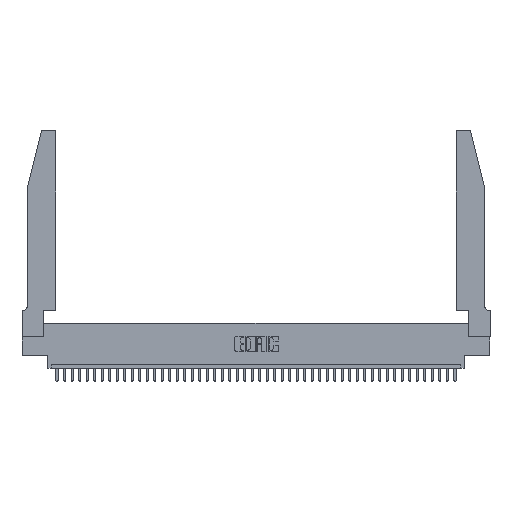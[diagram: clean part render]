
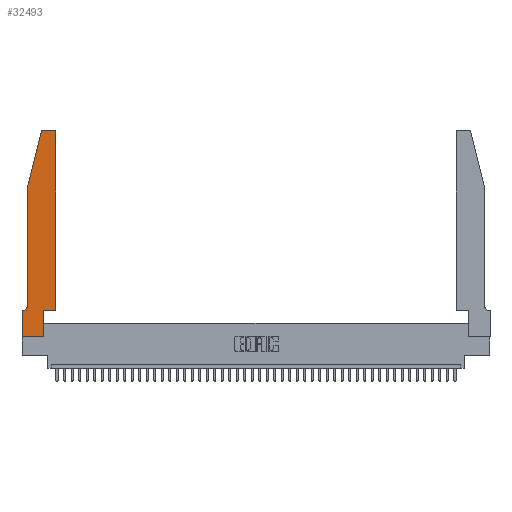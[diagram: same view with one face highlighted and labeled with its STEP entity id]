
A CAD part, top view. The second image highlights one B-rep face of the part: STEP entity #32493.
In plain terms, the highlighted planar face has unit normal (0, 0, 1).
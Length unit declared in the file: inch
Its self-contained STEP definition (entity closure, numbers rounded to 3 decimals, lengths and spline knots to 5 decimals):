
#1047 = CARTESIAN_POINT ( 'NONE',  ( 0.0755, 2., 0.37 ) ) ;
#1099 = VECTOR ( 'NONE', #38962, 39.37008 ) ;
#1119 = FACE_OUTER_BOUND ( 'NONE', #25102, .T. ) ;
#1411 = EDGE_CURVE ( 'NONE', #17696, #33769, #24357, .T. ) ;
#1927 = LINE ( 'NONE', #16082, #43422 ) ;
#2068 = VECTOR ( 'NONE', #18212, 39.37008 ) ;
#2736 = CIRCLE ( 'NONE', #26827, 0.03 ) ;
#2953 = VERTEX_POINT ( 'NONE', #4445 ) ;
#3896 = LINE ( 'NONE', #5352, #18376 ) ;
#4217 = EDGE_CURVE ( 'NONE', #33769, #29964, #24184, .T. ) ;
#4397 = EDGE_CURVE ( 'NONE', #36205, #2953, #17223, .T. ) ;
#4445 = CARTESIAN_POINT ( 'NONE',  ( 0.4205, 2.75, 0.37 ) ) ;
#4448 = DIRECTION ( 'NONE',  ( -1., 0., 0. ) ) ;
#4806 = CARTESIAN_POINT ( 'NONE',  ( 0., 0., 0.37 ) ) ;
#5143 = ORIENTED_EDGE ( 'NONE', *, *, #42124, .T. ) ;
#5352 = CARTESIAN_POINT ( 'NONE',  ( 0.4505, 0.35, 0.37 ) ) ;
#5891 = EDGE_CURVE ( 'NONE', #28611, #9246, #10174, .T. ) ;
#6174 = DIRECTION ( 'NONE',  ( 0., 1., 0. ) ) ;
#7845 = CARTESIAN_POINT ( 'NONE',  ( 0.4205, 2.72, 0.37 ) ) ;
#9045 = DIRECTION ( 'NONE',  ( 0., 0., 1. ) ) ;
#9246 = VERTEX_POINT ( 'NONE', #1047 ) ;
#9810 = AXIS2_PLACEMENT_3D ( 'NONE', #7845, #14760, #38531 ) ;
#10054 = ORIENTED_EDGE ( 'NONE', *, *, #1411, .T. ) ;
#10174 = LINE ( 'NONE', #28680, #30915 ) ;
#11114 = LINE ( 'NONE', #15453, #2068 ) ;
#11143 = CARTESIAN_POINT ( 'NONE',  ( 0., 0., 0.37 ) ) ;
#11722 = VECTOR ( 'NONE', #35917, 39.37008 ) ;
#14369 = DIRECTION ( 'NONE',  ( 1., 0., 0. ) ) ;
#14527 = AXIS2_PLACEMENT_3D ( 'NONE', #43108, #9045, #33290 ) ;
#14609 = ORIENTED_EDGE ( 'NONE', *, *, #4397, .T. ) ;
#14760 = DIRECTION ( 'NONE',  ( 0., 0., 1. ) ) ;
#15453 = CARTESIAN_POINT ( 'NONE',  ( 0., 0., 0.37 ) ) ;
#16082 = CARTESIAN_POINT ( 'NONE',  ( 0.2865, 0.35, 0.37 ) ) ;
#16674 = CARTESIAN_POINT ( 'NONE',  ( 0.0055, 0.35, 0.37 ) ) ;
#17223 = CIRCLE ( 'NONE', #9810, 0.03 ) ;
#17302 = EDGE_CURVE ( 'NONE', #2953, #28979, #42153, .T. ) ;
#17434 = ORIENTED_EDGE ( 'NONE', *, *, #34418, .T. ) ;
#17696 = VERTEX_POINT ( 'NONE', #31100 ) ;
#18212 = DIRECTION ( 'NONE',  ( 1., 0., 0. ) ) ;
#18376 = VECTOR ( 'NONE', #19092, 39.37008 ) ;
#19009 = DIRECTION ( 'NONE',  ( -1., 0., 0. ) ) ;
#19092 = DIRECTION ( 'NONE',  ( 0., 1., 0. ) ) ;
#19240 = EDGE_CURVE ( 'NONE', #21000, #33388, #11114, .T. ) ;
#19269 = VERTEX_POINT ( 'NONE', #37782 ) ;
#19767 = PLANE ( 'NONE',  #14527 ) ;
#20095 = CARTESIAN_POINT ( 'NONE',  ( 0.2865, 0.35, 0.37 ) ) ;
#20472 = DIRECTION ( 'NONE',  ( 1., 0., 0. ) ) ;
#20912 = CARTESIAN_POINT ( 'NONE',  ( 0.4505, 0.35, 0.37 ) ) ;
#21000 = VERTEX_POINT ( 'NONE', #4806 ) ;
#21328 = CARTESIAN_POINT ( 'NONE',  ( 0., 0.35, 0.37 ) ) ;
#22362 = CARTESIAN_POINT ( 'NONE',  ( 0.2605, 2.75, 0.37 ) ) ;
#22455 = CARTESIAN_POINT ( 'NONE',  ( 0.0755, 0.35, 0.37 ) ) ;
#23113 = ORIENTED_EDGE ( 'NONE', *, *, #42888, .T. ) ;
#23360 = VECTOR ( 'NONE', #14369, 39.37008 ) ;
#23473 = LINE ( 'NONE', #32483, #11722 ) ;
#23914 = CARTESIAN_POINT ( 'NONE',  ( 0.4505, 2.72, 0.37 ) ) ;
#24184 = LINE ( 'NONE', #22455, #42802 ) ;
#24357 = CIRCLE ( 'NONE', #38618, 0.07 ) ;
#24699 = CARTESIAN_POINT ( 'NONE',  ( 0.2865, 0., 0.37 ) ) ;
#24901 = CARTESIAN_POINT ( 'NONE',  ( 0.0055, 0.42, 0.37 ) ) ;
#25102 = EDGE_LOOP ( 'NONE', ( #42852, #31682, #36354, #23113, #10054, #36362, #5143, #40101, #42483, #17434, #35818, #14609 ) ) ;
#25788 = DIRECTION ( 'NONE',  ( -1., 0., 0. ) ) ;
#26827 = AXIS2_PLACEMENT_3D ( 'NONE', #43818, #40810, #20472 ) ;
#27795 = VECTOR ( 'NONE', #25788, 39.37008 ) ;
#28123 = CARTESIAN_POINT ( 'NONE',  ( 0.284, 2.75, 0.37 ) ) ;
#28611 = VERTEX_POINT ( 'NONE', #36499 ) ;
#28680 = CARTESIAN_POINT ( 'NONE',  ( 0.0755, 2., 0.37 ) ) ;
#28979 = VERTEX_POINT ( 'NONE', #28123 ) ;
#29964 = VERTEX_POINT ( 'NONE', #21328 ) ;
#30721 = LINE ( 'NONE', #20912, #23360 ) ;
#30915 = VECTOR ( 'NONE', #42482, 39.37008 ) ;
#31100 = CARTESIAN_POINT ( 'NONE',  ( 0.0755, 0.42, 0.37 ) ) ;
#31682 = ORIENTED_EDGE ( 'NONE', *, *, #32652, .T. ) ;
#32483 = CARTESIAN_POINT ( 'NONE',  ( 0.0755, 2., 0.37 ) ) ;
#32493 = ADVANCED_FACE ( 'NONE', ( #1119 ), #19767, .T. ) ;
#32652 = EDGE_CURVE ( 'NONE', #28979, #28611, #2736, .T. ) ;
#33290 = DIRECTION ( 'NONE',  ( 1., 0., 0. ) ) ;
#33388 = VERTEX_POINT ( 'NONE', #24699 ) ;
#33769 = VERTEX_POINT ( 'NONE', #16674 ) ;
#34124 = LINE ( 'NONE', #11143, #1099 ) ;
#34418 = EDGE_CURVE ( 'NONE', #42627, #19269, #30721, .T. ) ;
#35818 = ORIENTED_EDGE ( 'NONE', *, *, #36910, .T. ) ;
#35917 = DIRECTION ( 'NONE',  ( 0., -1., 0. ) ) ;
#36205 = VERTEX_POINT ( 'NONE', #23914 ) ;
#36354 = ORIENTED_EDGE ( 'NONE', *, *, #5891, .T. ) ;
#36362 = ORIENTED_EDGE ( 'NONE', *, *, #4217, .T. ) ;
#36499 = CARTESIAN_POINT ( 'NONE',  ( 0.25487, 2.72718, 0.37 ) ) ;
#36910 = EDGE_CURVE ( 'NONE', #19269, #36205, #3896, .T. ) ;
#37782 = CARTESIAN_POINT ( 'NONE',  ( 0.4505, 0.35, 0.37 ) ) ;
#38531 = DIRECTION ( 'NONE',  ( 1., 0., 0. ) ) ;
#38618 = AXIS2_PLACEMENT_3D ( 'NONE', #24901, #41384, #4448 ) ;
#38850 = EDGE_CURVE ( 'NONE', #33388, #42627, #1927, .T. ) ;
#38962 = DIRECTION ( 'NONE',  ( 0., -1., 0. ) ) ;
#40101 = ORIENTED_EDGE ( 'NONE', *, *, #19240, .T. ) ;
#40810 = DIRECTION ( 'NONE',  ( 0., 0., 1. ) ) ;
#41384 = DIRECTION ( 'NONE',  ( 0., 0., -1. ) ) ;
#42124 = EDGE_CURVE ( 'NONE', #29964, #21000, #34124, .T. ) ;
#42153 = LINE ( 'NONE', #22362, #27795 ) ;
#42482 = DIRECTION ( 'NONE',  ( -0.239, -0.971, 0. ) ) ;
#42483 = ORIENTED_EDGE ( 'NONE', *, *, #38850, .T. ) ;
#42627 = VERTEX_POINT ( 'NONE', #20095 ) ;
#42802 = VECTOR ( 'NONE', #19009, 39.37008 ) ;
#42852 = ORIENTED_EDGE ( 'NONE', *, *, #17302, .T. ) ;
#42888 = EDGE_CURVE ( 'NONE', #9246, #17696, #23473, .T. ) ;
#43108 = CARTESIAN_POINT ( 'NONE',  ( 0., 0.35, 0.37 ) ) ;
#43422 = VECTOR ( 'NONE', #6174, 39.37008 ) ;
#43818 = CARTESIAN_POINT ( 'NONE',  ( 0.284, 2.72, 0.37 ) ) ;
